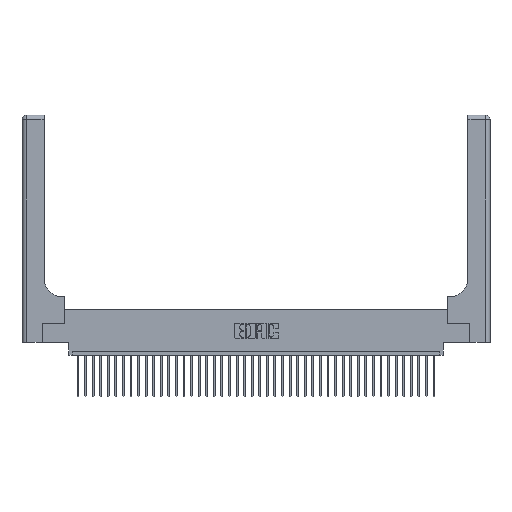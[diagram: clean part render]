
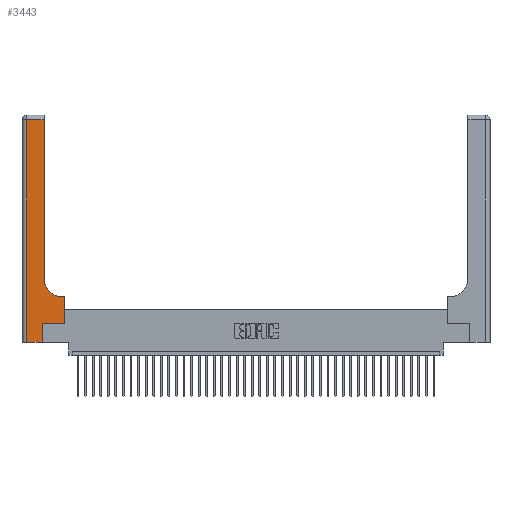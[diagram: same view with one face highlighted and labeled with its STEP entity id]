
A CAD part, top view. The second image highlights one B-rep face of the part: STEP entity #3443.
In plain terms, the highlighted planar face has unit normal (0, 0, 1).
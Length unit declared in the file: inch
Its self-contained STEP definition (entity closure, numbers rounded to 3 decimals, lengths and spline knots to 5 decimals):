
#536 = EDGE_CURVE ( 'NONE', #2508, #16624, #15467, .T. ) ;
#833 = CARTESIAN_POINT ( 'NONE',  ( 0.2915, 0.6, 0.37 ) ) ;
#1326 = CARTESIAN_POINT ( 'NONE',  ( 0.2915, 2.94, 0.37 ) ) ;
#2374 = AXIS2_PLACEMENT_3D ( 'NONE', #36863, #27519, #30672 ) ;
#2508 = VERTEX_POINT ( 'NONE', #39384 ) ;
#2665 = EDGE_CURVE ( 'NONE', #17422, #9244, #16934, .T. ) ;
#3443 = ADVANCED_FACE ( 'NONE', ( #31640 ), #5776, .F. ) ;
#3741 = DIRECTION ( 'NONE',  ( -1., 0., 0. ) ) ;
#4283 = EDGE_CURVE ( 'NONE', #40276, #39591, #31566, .T. ) ;
#4452 = DIRECTION ( 'NONE',  ( 0., 1., 0. ) ) ;
#4607 = CARTESIAN_POINT ( 'NONE',  ( 0.5585, 0.25, 0.37 ) ) ;
#4974 = DIRECTION ( 'NONE',  ( 0., 1., 0. ) ) ;
#5647 = DIRECTION ( 'NONE',  ( 0., 0., -1. ) ) ;
#5776 = PLANE ( 'NONE',  #18372 ) ;
#6604 = VECTOR ( 'NONE', #7914, 39.37008 ) ;
#7914 = DIRECTION ( 'NONE',  ( 0., 1., 0. ) ) ;
#8322 = CARTESIAN_POINT ( 'NONE',  ( 0.06, 2.94, 0.37 ) ) ;
#8541 = VERTEX_POINT ( 'NONE', #25027 ) ;
#8668 = CARTESIAN_POINT ( 'NONE',  ( 0.06, 3., 0.37 ) ) ;
#9244 = VERTEX_POINT ( 'NONE', #14279 ) ;
#9466 = LINE ( 'NONE', #36232, #12403 ) ;
#10044 = ORIENTED_EDGE ( 'NONE', *, *, #28266, .T. ) ;
#10595 = LINE ( 'NONE', #23191, #12103 ) ;
#12103 = VECTOR ( 'NONE', #4452, 39.37008 ) ;
#12403 = VECTOR ( 'NONE', #4974, 39.37008 ) ;
#12566 = ORIENTED_EDGE ( 'NONE', *, *, #19231, .T. ) ;
#12899 = CARTESIAN_POINT ( 'NONE',  ( 0.06, 0., 0.37 ) ) ;
#13332 = EDGE_CURVE ( 'NONE', #39591, #18230, #36679, .T. ) ;
#13824 = LINE ( 'NONE', #833, #32444 ) ;
#13842 = ORIENTED_EDGE ( 'NONE', *, *, #2665, .T. ) ;
#13952 = CARTESIAN_POINT ( 'NONE',  ( 0.269, 0.25, 0.37 ) ) ;
#14279 = CARTESIAN_POINT ( 'NONE',  ( 0.2915, 0.85, 0.37 ) ) ;
#14523 = ORIENTED_EDGE ( 'NONE', *, *, #536, .T. ) ;
#14608 = ORIENTED_EDGE ( 'NONE', *, *, #4283, .T. ) ;
#15467 = LINE ( 'NONE', #4607, #6604 ) ;
#16624 = VERTEX_POINT ( 'NONE', #33335 ) ;
#16934 = CIRCLE ( 'NONE', #2374, 0.25 ) ;
#17281 = DIRECTION ( 'NONE',  ( 1., 0., 0. ) ) ;
#17422 = VERTEX_POINT ( 'NONE', #19624 ) ;
#17499 = VECTOR ( 'NONE', #26886, 39.37008 ) ;
#18230 = VERTEX_POINT ( 'NONE', #12899 ) ;
#18372 = AXIS2_PLACEMENT_3D ( 'NONE', #27839, #5647, #24817 ) ;
#19099 = EDGE_CURVE ( 'NONE', #16624, #17422, #13824, .T. ) ;
#19231 = EDGE_CURVE ( 'NONE', #9244, #40276, #9466, .T. ) ;
#19624 = CARTESIAN_POINT ( 'NONE',  ( 0.5415, 0.6, 0.37 ) ) ;
#19991 = CARTESIAN_POINT ( 'NONE',  ( 0., 0., 0.37 ) ) ;
#20282 = VERTEX_POINT ( 'NONE', #28192 ) ;
#23191 = CARTESIAN_POINT ( 'NONE',  ( 0.269, 0., 0.37 ) ) ;
#23760 = VECTOR ( 'NONE', #17281, 39.37008 ) ;
#24817 = DIRECTION ( 'NONE',  ( -1., 0., 0. ) ) ;
#25027 = CARTESIAN_POINT ( 'NONE',  ( 0.269, 0.25, 0.37 ) ) ;
#26857 = DIRECTION ( 'NONE',  ( 1., 0., 0. ) ) ;
#26886 = DIRECTION ( 'NONE',  ( 0., -1., 0. ) ) ;
#27519 = DIRECTION ( 'NONE',  ( 0., 0., -1. ) ) ;
#27839 = CARTESIAN_POINT ( 'NONE',  ( 0., 3., 0.37 ) ) ;
#28065 = EDGE_LOOP ( 'NONE', ( #12566, #14608, #28207, #31556, #36139, #10044, #14523, #32976, #13842 ) ) ;
#28192 = CARTESIAN_POINT ( 'NONE',  ( 0.269, 0., 0.37 ) ) ;
#28207 = ORIENTED_EDGE ( 'NONE', *, *, #13332, .T. ) ;
#28266 = EDGE_CURVE ( 'NONE', #8541, #2508, #33730, .T. ) ;
#30109 = EDGE_CURVE ( 'NONE', #18230, #20282, #38987, .T. ) ;
#30672 = DIRECTION ( 'NONE',  ( 1., 0., 0. ) ) ;
#31556 = ORIENTED_EDGE ( 'NONE', *, *, #30109, .T. ) ;
#31566 = LINE ( 'NONE', #39709, #36534 ) ;
#31640 = FACE_OUTER_BOUND ( 'NONE', #28065, .T. ) ;
#31655 = EDGE_CURVE ( 'NONE', #20282, #8541, #10595, .T. ) ;
#32444 = VECTOR ( 'NONE', #3741, 39.37008 ) ;
#32976 = ORIENTED_EDGE ( 'NONE', *, *, #19099, .T. ) ;
#33208 = DIRECTION ( 'NONE',  ( -1., 0., 0. ) ) ;
#33335 = CARTESIAN_POINT ( 'NONE',  ( 0.5585, 0.6, 0.37 ) ) ;
#33730 = LINE ( 'NONE', #13952, #39161 ) ;
#36139 = ORIENTED_EDGE ( 'NONE', *, *, #31655, .T. ) ;
#36232 = CARTESIAN_POINT ( 'NONE',  ( 0.2915, 3., 0.37 ) ) ;
#36534 = VECTOR ( 'NONE', #33208, 39.37008 ) ;
#36679 = LINE ( 'NONE', #8668, #17499 ) ;
#36863 = CARTESIAN_POINT ( 'NONE',  ( 0.5415, 0.85, 0.37 ) ) ;
#38987 = LINE ( 'NONE', #19991, #23760 ) ;
#39161 = VECTOR ( 'NONE', #26857, 39.37008 ) ;
#39384 = CARTESIAN_POINT ( 'NONE',  ( 0.5585, 0.25, 0.37 ) ) ;
#39591 = VERTEX_POINT ( 'NONE', #8322 ) ;
#39709 = CARTESIAN_POINT ( 'NONE',  ( 0., 2.94, 0.37 ) ) ;
#40276 = VERTEX_POINT ( 'NONE', #1326 ) ;
